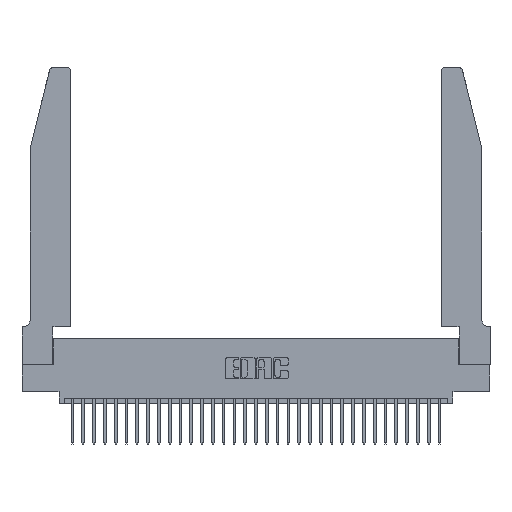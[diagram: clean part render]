
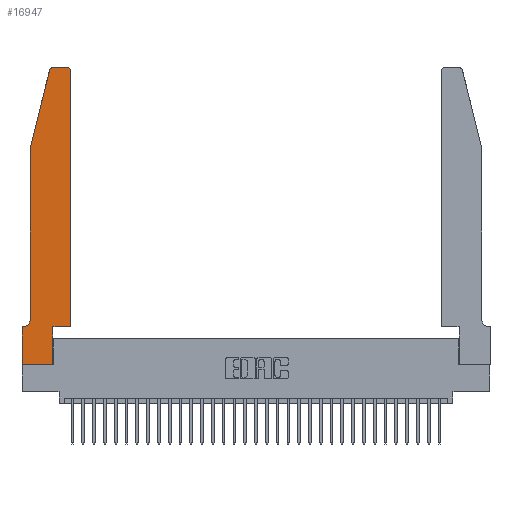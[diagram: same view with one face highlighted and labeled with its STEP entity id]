
A CAD part, top view. The second image highlights one B-rep face of the part: STEP entity #16947.
In plain terms, the highlighted planar face has unit normal (0, 0, 1).
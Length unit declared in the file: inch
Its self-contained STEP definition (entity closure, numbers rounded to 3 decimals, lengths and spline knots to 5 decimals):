
#388 = CARTESIAN_POINT ( 'NONE',  ( 0.25487, 2.72718, 0.37 ) ) ;
#683 = LINE ( 'NONE', #17668, #7655 ) ;
#1186 = EDGE_LOOP ( 'NONE', ( #17508, #3989, #28121, #20831, #30802, #8618, #16423, #29540, #8160, #3188, #3519, #28461 ) ) ;
#1243 = DIRECTION ( 'NONE',  ( -1., 0., 0. ) ) ;
#1373 = VERTEX_POINT ( 'NONE', #9064 ) ;
#1685 = DIRECTION ( 'NONE',  ( 0., 0., 1. ) ) ;
#2430 = VECTOR ( 'NONE', #17022, 39.37008 ) ;
#2602 = CARTESIAN_POINT ( 'NONE',  ( 0., 0., 0.37 ) ) ;
#2882 = VERTEX_POINT ( 'NONE', #4073 ) ;
#3188 = ORIENTED_EDGE ( 'NONE', *, *, #8338, .T. ) ;
#3519 = ORIENTED_EDGE ( 'NONE', *, *, #13998, .T. ) ;
#3989 = ORIENTED_EDGE ( 'NONE', *, *, #25851, .T. ) ;
#4073 = CARTESIAN_POINT ( 'NONE',  ( 0.284, 2.75, 0.37 ) ) ;
#4647 = CIRCLE ( 'NONE', #15148, 0.03 ) ;
#4696 = VECTOR ( 'NONE', #1243, 39.37008 ) ;
#5761 = CARTESIAN_POINT ( 'NONE',  ( 0.0055, 0.35, 0.37 ) ) ;
#7022 = DIRECTION ( 'NONE',  ( 0., 0., -1. ) ) ;
#7248 = CARTESIAN_POINT ( 'NONE',  ( 0.2865, 0., 0.37 ) ) ;
#7655 = VECTOR ( 'NONE', #25350, 39.37008 ) ;
#8112 = CIRCLE ( 'NONE', #29246, 0.03 ) ;
#8160 = ORIENTED_EDGE ( 'NONE', *, *, #10102, .T. ) ;
#8281 = VERTEX_POINT ( 'NONE', #5761 ) ;
#8338 = EDGE_CURVE ( 'NONE', #20507, #21765, #17736, .T. ) ;
#8618 = ORIENTED_EDGE ( 'NONE', *, *, #25301, .T. ) ;
#8952 = DIRECTION ( 'NONE',  ( 0., -1., 0. ) ) ;
#9064 = CARTESIAN_POINT ( 'NONE',  ( 0.0755, 0.42, 0.37 ) ) ;
#10102 = EDGE_CURVE ( 'NONE', #10304, #20507, #23241, .T. ) ;
#10304 = VERTEX_POINT ( 'NONE', #7248 ) ;
#10643 = VECTOR ( 'NONE', #28010, 39.37008 ) ;
#10676 = CARTESIAN_POINT ( 'NONE',  ( 0.4505, 0.35, 0.37 ) ) ;
#10814 = VECTOR ( 'NONE', #19794, 39.37008 ) ;
#11099 = CARTESIAN_POINT ( 'NONE',  ( 0.4505, 0.35, 0.37 ) ) ;
#11262 = CARTESIAN_POINT ( 'NONE',  ( 0.0755, 2., 0.37 ) ) ;
#11720 = LINE ( 'NONE', #14365, #4696 ) ;
#11834 = CIRCLE ( 'NONE', #18047, 0.07 ) ;
#12371 = VERTEX_POINT ( 'NONE', #20162 ) ;
#12911 = CARTESIAN_POINT ( 'NONE',  ( 0.2865, 0.35, 0.37 ) ) ;
#13599 = EDGE_CURVE ( 'NONE', #21923, #2882, #11720, .T. ) ;
#13626 = LINE ( 'NONE', #11262, #33031 ) ;
#13815 = DIRECTION ( 'NONE',  ( 0., 0., 1. ) ) ;
#13998 = EDGE_CURVE ( 'NONE', #21765, #27329, #28538, .T. ) ;
#14258 = CARTESIAN_POINT ( 'NONE',  ( 0., 0., 0.37 ) ) ;
#14365 = CARTESIAN_POINT ( 'NONE',  ( 0.2605, 2.75, 0.37 ) ) ;
#14422 = CARTESIAN_POINT ( 'NONE',  ( 0.2865, 0.35, 0.37 ) ) ;
#14975 = CARTESIAN_POINT ( 'NONE',  ( 0.4205, 2.72, 0.37 ) ) ;
#15148 = AXIS2_PLACEMENT_3D ( 'NONE', #14975, #32680, #17574 ) ;
#15227 = EDGE_CURVE ( 'NONE', #12371, #24096, #23708, .T. ) ;
#15327 = CARTESIAN_POINT ( 'NONE',  ( 0.0755, 0.35, 0.37 ) ) ;
#16065 = FACE_OUTER_BOUND ( 'NONE', #1186, .T. ) ;
#16423 = ORIENTED_EDGE ( 'NONE', *, *, #15227, .T. ) ;
#16442 = DIRECTION ( 'NONE',  ( -0.239, -0.971, 0. ) ) ;
#16906 = VECTOR ( 'NONE', #8952, 39.37008 ) ;
#16947 = ADVANCED_FACE ( 'NONE', ( #16065 ), #24002, .T. ) ;
#17012 = EDGE_CURVE ( 'NONE', #24303, #1373, #13626, .T. ) ;
#17022 = DIRECTION ( 'NONE',  ( 0., 1., 0. ) ) ;
#17420 = CARTESIAN_POINT ( 'NONE',  ( 0.284, 2.72, 0.37 ) ) ;
#17508 = ORIENTED_EDGE ( 'NONE', *, *, #13599, .T. ) ;
#17574 = DIRECTION ( 'NONE',  ( 1., 0., 0. ) ) ;
#17668 = CARTESIAN_POINT ( 'NONE',  ( 0., 0., 0.37 ) ) ;
#17736 = LINE ( 'NONE', #24934, #10814 ) ;
#18047 = AXIS2_PLACEMENT_3D ( 'NONE', #22646, #7022, #25160 ) ;
#18506 = DIRECTION ( 'NONE',  ( 0., 1., 0. ) ) ;
#18669 = VERTEX_POINT ( 'NONE', #388 ) ;
#19074 = EDGE_CURVE ( 'NONE', #24096, #10304, #683, .T. ) ;
#19794 = DIRECTION ( 'NONE',  ( 1., 0., 0. ) ) ;
#19980 = DIRECTION ( 'NONE',  ( 1., 0., 0. ) ) ;
#20162 = CARTESIAN_POINT ( 'NONE',  ( 0., 0.35, 0.37 ) ) ;
#20507 = VERTEX_POINT ( 'NONE', #12911 ) ;
#20831 = ORIENTED_EDGE ( 'NONE', *, *, #17012, .T. ) ;
#21765 = VERTEX_POINT ( 'NONE', #11099 ) ;
#21923 = VERTEX_POINT ( 'NONE', #24495 ) ;
#22102 = EDGE_CURVE ( 'NONE', #27329, #21923, #4647, .T. ) ;
#22646 = CARTESIAN_POINT ( 'NONE',  ( 0.0055, 0.42, 0.37 ) ) ;
#23241 = LINE ( 'NONE', #14422, #2430 ) ;
#23575 = LINE ( 'NONE', #15327, #10643 ) ;
#23708 = LINE ( 'NONE', #14258, #16906 ) ;
#24002 = PLANE ( 'NONE',  #31312 ) ;
#24096 = VERTEX_POINT ( 'NONE', #2602 ) ;
#24303 = VERTEX_POINT ( 'NONE', #29249 ) ;
#24495 = CARTESIAN_POINT ( 'NONE',  ( 0.4205, 2.75, 0.37 ) ) ;
#24934 = CARTESIAN_POINT ( 'NONE',  ( 0.4505, 0.35, 0.37 ) ) ;
#25160 = DIRECTION ( 'NONE',  ( -1., 0., 0. ) ) ;
#25301 = EDGE_CURVE ( 'NONE', #8281, #12371, #23575, .T. ) ;
#25350 = DIRECTION ( 'NONE',  ( 1., 0., 0. ) ) ;
#25851 = EDGE_CURVE ( 'NONE', #2882, #18669, #8112, .T. ) ;
#26971 = VECTOR ( 'NONE', #18506, 39.37008 ) ;
#27329 = VERTEX_POINT ( 'NONE', #31552 ) ;
#27996 = LINE ( 'NONE', #29073, #28778 ) ;
#28010 = DIRECTION ( 'NONE',  ( -1., 0., 0. ) ) ;
#28121 = ORIENTED_EDGE ( 'NONE', *, *, #32768, .T. ) ;
#28205 = EDGE_CURVE ( 'NONE', #1373, #8281, #11834, .T. ) ;
#28461 = ORIENTED_EDGE ( 'NONE', *, *, #22102, .T. ) ;
#28538 = LINE ( 'NONE', #10676, #26971 ) ;
#28778 = VECTOR ( 'NONE', #16442, 39.37008 ) ;
#29073 = CARTESIAN_POINT ( 'NONE',  ( 0.0755, 2., 0.37 ) ) ;
#29246 = AXIS2_PLACEMENT_3D ( 'NONE', #17420, #1685, #19980 ) ;
#29249 = CARTESIAN_POINT ( 'NONE',  ( 0.0755, 2., 0.37 ) ) ;
#29259 = DIRECTION ( 'NONE',  ( 0., -1., 0. ) ) ;
#29540 = ORIENTED_EDGE ( 'NONE', *, *, #19074, .T. ) ;
#30802 = ORIENTED_EDGE ( 'NONE', *, *, #28205, .T. ) ;
#31312 = AXIS2_PLACEMENT_3D ( 'NONE', #31332, #13815, #31559 ) ;
#31332 = CARTESIAN_POINT ( 'NONE',  ( 0., 0.35, 0.37 ) ) ;
#31552 = CARTESIAN_POINT ( 'NONE',  ( 0.4505, 2.72, 0.37 ) ) ;
#31559 = DIRECTION ( 'NONE',  ( 1., 0., 0. ) ) ;
#32680 = DIRECTION ( 'NONE',  ( 0., 0., 1. ) ) ;
#32768 = EDGE_CURVE ( 'NONE', #18669, #24303, #27996, .T. ) ;
#33031 = VECTOR ( 'NONE', #29259, 39.37008 ) ;
